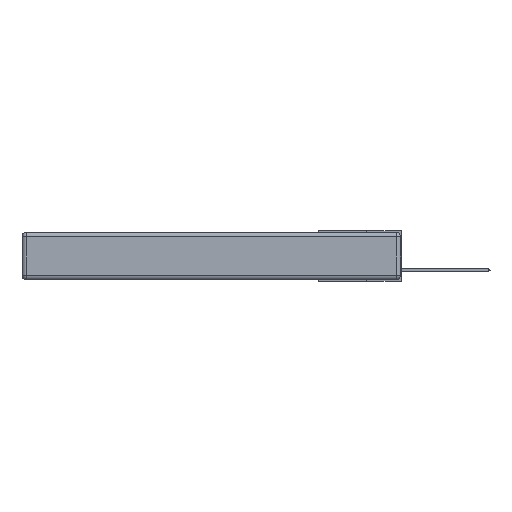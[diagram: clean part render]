
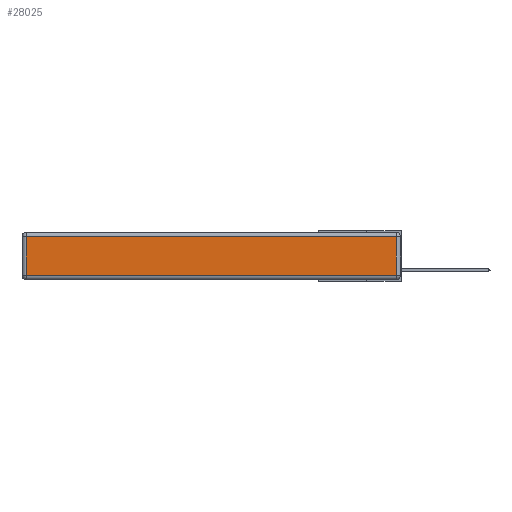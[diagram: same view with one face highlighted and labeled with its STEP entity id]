
A CAD part, left-side view. The second image highlights one B-rep face of the part: STEP entity #28025.
In plain terms, the highlighted planar face has unit normal (-1, 0, 0).
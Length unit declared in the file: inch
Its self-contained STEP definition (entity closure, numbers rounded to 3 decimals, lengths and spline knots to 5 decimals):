
#51 = EDGE_CURVE ( 'NONE', #15456, #25475, #4361, .T. ) ;
#1294 = DIRECTION ( 'NONE',  ( -1., 0., 0. ) ) ;
#3023 = CARTESIAN_POINT ( 'NONE',  ( 0., 0.03, -0.03 ) ) ;
#3597 = CARTESIAN_POINT ( 'NONE',  ( 0., 0.03, -0.313 ) ) ;
#4361 = LINE ( 'NONE', #27488, #6246 ) ;
#6246 = VECTOR ( 'NONE', #17860, 39.37008 ) ;
#6963 = ORIENTED_EDGE ( 'NONE', *, *, #29135, .T. ) ;
#7694 = EDGE_LOOP ( 'NONE', ( #6963, #27826, #19482, #7913 ) ) ;
#7913 = ORIENTED_EDGE ( 'NONE', *, *, #51, .T. ) ;
#8018 = CARTESIAN_POINT ( 'NONE',  ( 0., 2.72, -0.03 ) ) ;
#9160 = DIRECTION ( 'NONE',  ( 0., 1., 0. ) ) ;
#10158 = LINE ( 'NONE', #29996, #22118 ) ;
#10732 = DIRECTION ( 'NONE',  ( 0., -1., 0. ) ) ;
#10975 = CARTESIAN_POINT ( 'NONE',  ( 0., 0., -0.343 ) ) ;
#11140 = CARTESIAN_POINT ( 'NONE',  ( 0., 2.75, -0.03 ) ) ;
#14948 = VERTEX_POINT ( 'NONE', #3597 ) ;
#15456 = VERTEX_POINT ( 'NONE', #8018 ) ;
#17860 = DIRECTION ( 'NONE',  ( 0., 0., -1. ) ) ;
#18565 = LINE ( 'NONE', #11140, #27517 ) ;
#19482 = ORIENTED_EDGE ( 'NONE', *, *, #26366, .T. ) ;
#19742 = DIRECTION ( 'NONE',  ( 0., 0., 1. ) ) ;
#19847 = VECTOR ( 'NONE', #19742, 39.37008 ) ;
#20612 = PLANE ( 'NONE',  #26763 ) ;
#22118 = VECTOR ( 'NONE', #10732, 39.37008 ) ;
#23166 = EDGE_CURVE ( 'NONE', #14948, #29973, #25808, .T. ) ;
#25475 = VERTEX_POINT ( 'NONE', #28741 ) ;
#25808 = LINE ( 'NONE', #29562, #19847 ) ;
#26366 = EDGE_CURVE ( 'NONE', #29973, #15456, #18565, .T. ) ;
#26763 = AXIS2_PLACEMENT_3D ( 'NONE', #10975, #1294, #30026 ) ;
#27430 = FACE_OUTER_BOUND ( 'NONE', #7694, .T. ) ;
#27488 = CARTESIAN_POINT ( 'NONE',  ( 0., 2.72, -0.343 ) ) ;
#27517 = VECTOR ( 'NONE', #9160, 39.37008 ) ;
#27826 = ORIENTED_EDGE ( 'NONE', *, *, #23166, .T. ) ;
#28025 = ADVANCED_FACE ( 'NONE', ( #27430 ), #20612, .T. ) ;
#28741 = CARTESIAN_POINT ( 'NONE',  ( 0., 2.72, -0.313 ) ) ;
#29135 = EDGE_CURVE ( 'NONE', #25475, #14948, #10158, .T. ) ;
#29562 = CARTESIAN_POINT ( 'NONE',  ( 0., 0.03, -0.343 ) ) ;
#29973 = VERTEX_POINT ( 'NONE', #3023 ) ;
#29996 = CARTESIAN_POINT ( 'NONE',  ( 0., 0., -0.313 ) ) ;
#30026 = DIRECTION ( 'NONE',  ( 0., 0., 1. ) ) ;
